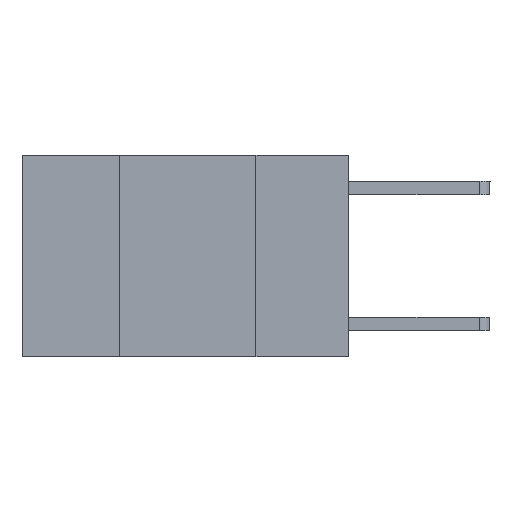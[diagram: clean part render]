
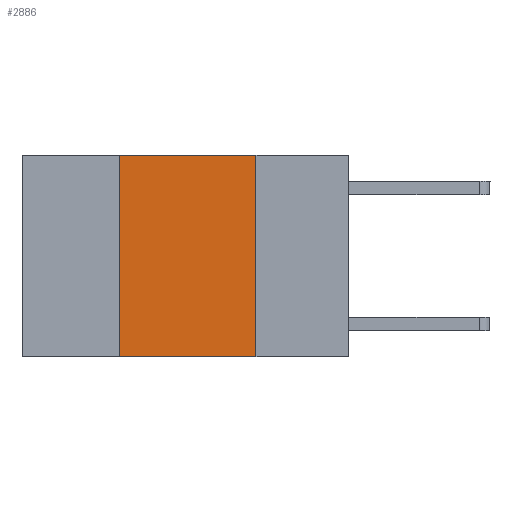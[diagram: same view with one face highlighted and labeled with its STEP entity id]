
A CAD part, left-side view. The second image highlights one B-rep face of the part: STEP entity #2886.
In plain terms, the highlighted planar face has unit normal (-1, 0, 0).
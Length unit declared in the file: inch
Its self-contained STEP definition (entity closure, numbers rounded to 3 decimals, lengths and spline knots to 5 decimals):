
#258 = VECTOR ( 'NONE', #2159, 39.37008 ) ;
#371 = CARTESIAN_POINT ( 'NONE',  ( 0., 0.42, 0. ) ) ;
#411 = VECTOR ( 'NONE', #6558, 39.37008 ) ;
#837 = PLANE ( 'NONE',  #8864 ) ;
#915 = DIRECTION ( 'NONE',  ( 0., 0., -1. ) ) ;
#1025 = VECTOR ( 'NONE', #6813, 39.37008 ) ;
#1187 = ORIENTED_EDGE ( 'NONE', *, *, #2735, .F. ) ;
#1557 = CARTESIAN_POINT ( 'NONE',  ( 0., 0.17, 0. ) ) ;
#1606 = EDGE_LOOP ( 'NONE', ( #5829, #2871, #1187, #8806 ) ) ;
#1886 = EDGE_CURVE ( 'NONE', #2532, #2875, #6508, .T. ) ;
#2159 = DIRECTION ( 'NONE',  ( 0., 0., 1. ) ) ;
#2335 = EDGE_CURVE ( 'NONE', #7865, #3419, #6677, .T. ) ;
#2532 = VERTEX_POINT ( 'NONE', #371 ) ;
#2735 = EDGE_CURVE ( 'NONE', #7865, #2532, #7860, .T. ) ;
#2871 = ORIENTED_EDGE ( 'NONE', *, *, #1886, .F. ) ;
#2875 = VERTEX_POINT ( 'NONE', #1557 ) ;
#2886 = ADVANCED_FACE ( 'NONE', ( #4449 ), #837, .F. ) ;
#2999 = DIRECTION ( 'NONE',  ( 0., 0., -1. ) ) ;
#3078 = LINE ( 'NONE', #8906, #5919 ) ;
#3098 = CARTESIAN_POINT ( 'NONE',  ( 0., 0.6, -0.37 ) ) ;
#3419 = VERTEX_POINT ( 'NONE', #5477 ) ;
#3722 = CARTESIAN_POINT ( 'NONE',  ( 0., 0.6, 0. ) ) ;
#4449 = FACE_OUTER_BOUND ( 'NONE', #1606, .T. ) ;
#5368 = EDGE_CURVE ( 'NONE', #2875, #3419, #3078, .T. ) ;
#5477 = CARTESIAN_POINT ( 'NONE',  ( 0., 0.17, -0.37 ) ) ;
#5587 = CARTESIAN_POINT ( 'NONE',  ( 0., 0.42, -0.37 ) ) ;
#5706 = CARTESIAN_POINT ( 'NONE',  ( 0., 0.6, 0. ) ) ;
#5728 = CARTESIAN_POINT ( 'NONE',  ( 0., 0.42, 0. ) ) ;
#5829 = ORIENTED_EDGE ( 'NONE', *, *, #5368, .F. ) ;
#5919 = VECTOR ( 'NONE', #915, 39.37008 ) ;
#6508 = LINE ( 'NONE', #5706, #411 ) ;
#6558 = DIRECTION ( 'NONE',  ( 0., -1., 0. ) ) ;
#6613 = DIRECTION ( 'NONE',  ( 1., 0., 0. ) ) ;
#6677 = LINE ( 'NONE', #3098, #1025 ) ;
#6813 = DIRECTION ( 'NONE',  ( 0., -1., 0. ) ) ;
#7860 = LINE ( 'NONE', #5728, #258 ) ;
#7865 = VERTEX_POINT ( 'NONE', #5587 ) ;
#8806 = ORIENTED_EDGE ( 'NONE', *, *, #2335, .T. ) ;
#8864 = AXIS2_PLACEMENT_3D ( 'NONE', #3722, #6613, #2999 ) ;
#8906 = CARTESIAN_POINT ( 'NONE',  ( 0., 0.17, 0. ) ) ;
